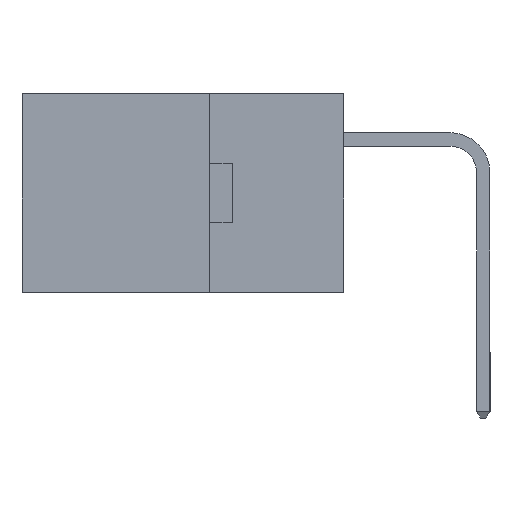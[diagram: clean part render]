
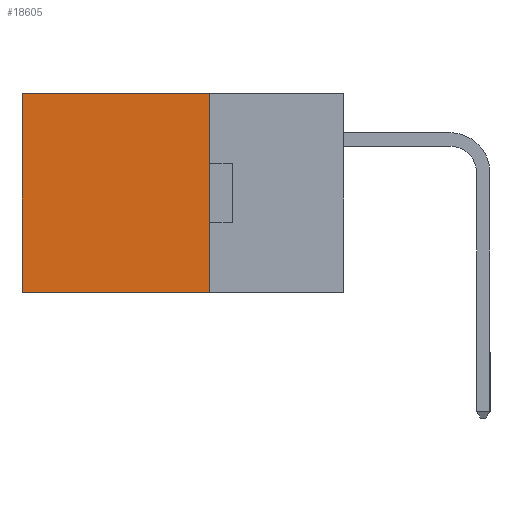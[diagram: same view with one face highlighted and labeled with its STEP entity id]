
A CAD part, left-side view. The second image highlights one B-rep face of the part: STEP entity #18605.
In plain terms, the highlighted planar face has unit normal (-1, 0, 0).
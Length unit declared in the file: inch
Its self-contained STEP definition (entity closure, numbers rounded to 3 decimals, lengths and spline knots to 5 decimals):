
#234 = CARTESIAN_POINT ( 'NONE',  ( 0.2615, 0.25, 0. ) ) ;
#2855 = CARTESIAN_POINT ( 'NONE',  ( 0.2615, 0.25, -0.37 ) ) ;
#4210 = EDGE_CURVE ( 'NONE', #11394, #24435, #21550, .T. ) ;
#6840 = VECTOR ( 'NONE', #23438, 39.37008 ) ;
#8304 = ORIENTED_EDGE ( 'NONE', *, *, #27229, .F. ) ;
#8360 = LINE ( 'NONE', #20895, #19338 ) ;
#8608 = CARTESIAN_POINT ( 'NONE',  ( 0.2615, 0.6, -0.37 ) ) ;
#10366 = LINE ( 'NONE', #24702, #22410 ) ;
#11394 = VERTEX_POINT ( 'NONE', #17830 ) ;
#11890 = EDGE_CURVE ( 'NONE', #25201, #24435, #10366, .T. ) ;
#12052 = EDGE_CURVE ( 'NONE', #14555, #11394, #25787, .T. ) ;
#12088 = DIRECTION ( 'NONE',  ( 1., 0., 0. ) ) ;
#12508 = ORIENTED_EDGE ( 'NONE', *, *, #12052, .T. ) ;
#12868 = ORIENTED_EDGE ( 'NONE', *, *, #4210, .T. ) ;
#13986 = DIRECTION ( 'NONE',  ( 0., 1., 0. ) ) ;
#14166 = PLANE ( 'NONE',  #20402 ) ;
#14404 = CARTESIAN_POINT ( 'NONE',  ( 0.2615, 0.6, -0.37 ) ) ;
#14555 = VERTEX_POINT ( 'NONE', #20344 ) ;
#17082 = ORIENTED_EDGE ( 'NONE', *, *, #11890, .F. ) ;
#17830 = CARTESIAN_POINT ( 'NONE',  ( 0.2615, 0.6, 0. ) ) ;
#18098 = FACE_OUTER_BOUND ( 'NONE', #20404, .T. ) ;
#18605 = ADVANCED_FACE ( 'NONE', ( #18098 ), #14166, .F. ) ;
#18630 = VECTOR ( 'NONE', #25690, 39.37008 ) ;
#19338 = VECTOR ( 'NONE', #25051, 39.37008 ) ;
#20344 = CARTESIAN_POINT ( 'NONE',  ( 0.2615, 0.25, 0. ) ) ;
#20402 = AXIS2_PLACEMENT_3D ( 'NONE', #22685, #12088, #20471 ) ;
#20404 = EDGE_LOOP ( 'NONE', ( #12868, #17082, #8304, #12508 ) ) ;
#20471 = DIRECTION ( 'NONE',  ( 0., 0., -1. ) ) ;
#20895 = CARTESIAN_POINT ( 'NONE',  ( 0.2615, 0.25, -0.37 ) ) ;
#21550 = LINE ( 'NONE', #8608, #18630 ) ;
#22410 = VECTOR ( 'NONE', #13986, 39.37008 ) ;
#22685 = CARTESIAN_POINT ( 'NONE',  ( 0.2615, 0.25, -0.37 ) ) ;
#23438 = DIRECTION ( 'NONE',  ( 0., 1., 0. ) ) ;
#24435 = VERTEX_POINT ( 'NONE', #14404 ) ;
#24702 = CARTESIAN_POINT ( 'NONE',  ( 0.2615, 0.25, -0.37 ) ) ;
#25051 = DIRECTION ( 'NONE',  ( 0., 0., -1. ) ) ;
#25201 = VERTEX_POINT ( 'NONE', #2855 ) ;
#25690 = DIRECTION ( 'NONE',  ( 0., 0., -1. ) ) ;
#25787 = LINE ( 'NONE', #234, #6840 ) ;
#27229 = EDGE_CURVE ( 'NONE', #14555, #25201, #8360, .T. ) ;
